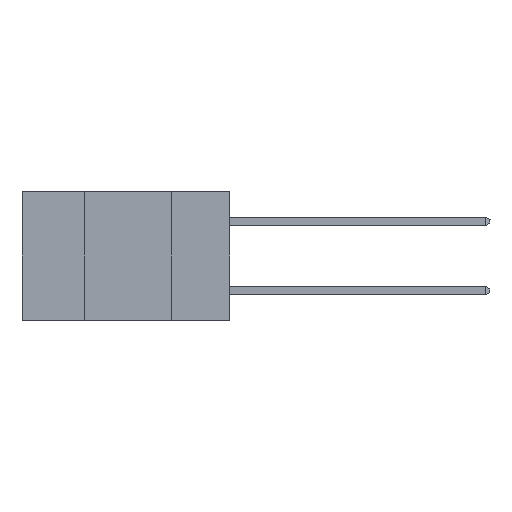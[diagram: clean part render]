
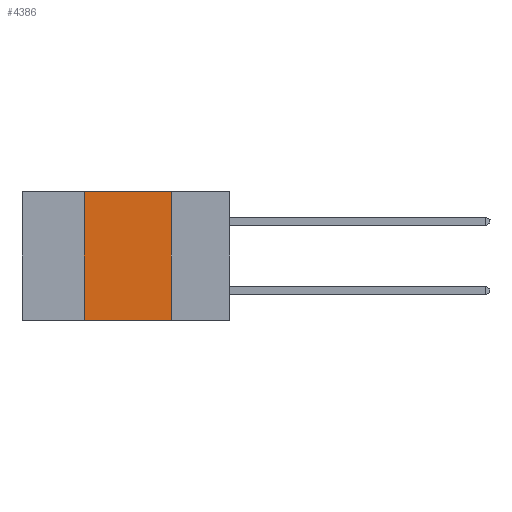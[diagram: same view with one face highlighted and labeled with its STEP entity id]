
A CAD part, left-side view. The second image highlights one B-rep face of the part: STEP entity #4386.
In plain terms, the highlighted planar face has unit normal (-1, 0, 0).
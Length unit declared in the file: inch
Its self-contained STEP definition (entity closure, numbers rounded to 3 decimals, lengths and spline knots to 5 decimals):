
#945 = LINE ( 'NONE', #11377, #5016 ) ;
#1041 = DIRECTION ( 'NONE',  ( 0., -1., 0. ) ) ;
#1151 = ORIENTED_EDGE ( 'NONE', *, *, #8379, .F. ) ;
#1162 = DIRECTION ( 'NONE',  ( 0., 0., 1. ) ) ;
#1556 = LINE ( 'NONE', #2078, #11306 ) ;
#2078 = CARTESIAN_POINT ( 'NONE',  ( 0., 0.6, 0. ) ) ;
#2094 = CARTESIAN_POINT ( 'NONE',  ( 0., 0.42, -0.37 ) ) ;
#2384 = CARTESIAN_POINT ( 'NONE',  ( 0., 0.42, 0. ) ) ;
#2542 = AXIS2_PLACEMENT_3D ( 'NONE', #2698, #6465, #12058 ) ;
#2698 = CARTESIAN_POINT ( 'NONE',  ( 0., 0.6, 0. ) ) ;
#2834 = VERTEX_POINT ( 'NONE', #2094 ) ;
#3452 = EDGE_CURVE ( 'NONE', #10591, #10471, #1556, .T. ) ;
#4312 = CARTESIAN_POINT ( 'NONE',  ( 0., 0.17, -0.37 ) ) ;
#4386 = ADVANCED_FACE ( 'NONE', ( #9408 ), #4532, .F. ) ;
#4532 = PLANE ( 'NONE',  #2542 ) ;
#4868 = VERTEX_POINT ( 'NONE', #4312 ) ;
#5016 = VECTOR ( 'NONE', #1162, 39.37008 ) ;
#5166 = EDGE_CURVE ( 'NONE', #2834, #10591, #945, .T. ) ;
#5406 = ORIENTED_EDGE ( 'NONE', *, *, #5166, .F. ) ;
#5657 = CARTESIAN_POINT ( 'NONE',  ( 0., 0.6, -0.37 ) ) ;
#5814 = CARTESIAN_POINT ( 'NONE',  ( 0., 0.17, 0. ) ) ;
#6465 = DIRECTION ( 'NONE',  ( 1., 0., 0. ) ) ;
#6657 = EDGE_CURVE ( 'NONE', #2834, #4868, #7626, .T. ) ;
#6963 = CARTESIAN_POINT ( 'NONE',  ( 0., 0.17, 0. ) ) ;
#7626 = LINE ( 'NONE', #5657, #9217 ) ;
#8288 = LINE ( 'NONE', #6963, #10047 ) ;
#8379 = EDGE_CURVE ( 'NONE', #10471, #4868, #8288, .T. ) ;
#9217 = VECTOR ( 'NONE', #1041, 39.37008 ) ;
#9408 = FACE_OUTER_BOUND ( 'NONE', #11928, .T. ) ;
#9497 = DIRECTION ( 'NONE',  ( 0., -1., 0. ) ) ;
#9674 = DIRECTION ( 'NONE',  ( 0., 0., -1. ) ) ;
#9699 = ORIENTED_EDGE ( 'NONE', *, *, #3452, .F. ) ;
#10047 = VECTOR ( 'NONE', #9674, 39.37008 ) ;
#10471 = VERTEX_POINT ( 'NONE', #5814 ) ;
#10591 = VERTEX_POINT ( 'NONE', #2384 ) ;
#11030 = ORIENTED_EDGE ( 'NONE', *, *, #6657, .T. ) ;
#11306 = VECTOR ( 'NONE', #9497, 39.37008 ) ;
#11377 = CARTESIAN_POINT ( 'NONE',  ( 0., 0.42, 0. ) ) ;
#11928 = EDGE_LOOP ( 'NONE', ( #1151, #9699, #5406, #11030 ) ) ;
#12058 = DIRECTION ( 'NONE',  ( 0., 0., -1. ) ) ;
